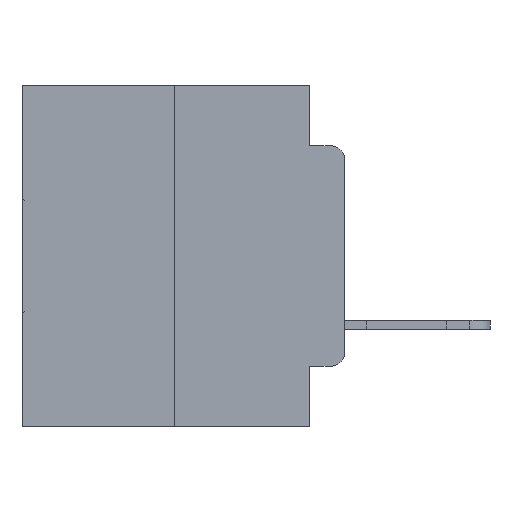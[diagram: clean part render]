
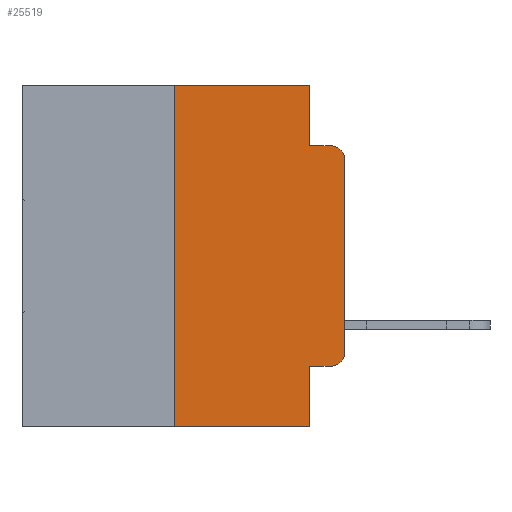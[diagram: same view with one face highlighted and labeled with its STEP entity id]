
A CAD part, left-side view. The second image highlights one B-rep face of the part: STEP entity #25519.
In plain terms, the highlighted planar face has unit normal (-1, 0, 0).
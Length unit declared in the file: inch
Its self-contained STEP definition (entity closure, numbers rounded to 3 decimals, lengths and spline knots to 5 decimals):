
#368 = LINE ( 'NONE', #13695, #17627 ) ;
#556 = VERTEX_POINT ( 'NONE', #14851 ) ;
#1905 = DIRECTION ( 'NONE',  ( 0., 0., 1. ) ) ;
#1913 = DIRECTION ( 'NONE',  ( -1., 0., 0. ) ) ;
#2659 = CARTESIAN_POINT ( 'NONE',  ( 0., 0.473, -0.5 ) ) ;
#3239 = PLANE ( 'NONE',  #23202 ) ;
#3346 = LINE ( 'NONE', #11373, #20342 ) ;
#3619 = CARTESIAN_POINT ( 'NONE',  ( 0., 0.02, -0.0885 ) ) ;
#3624 = EDGE_CURVE ( 'NONE', #8612, #556, #3346, .T. ) ;
#4244 = AXIS2_PLACEMENT_3D ( 'NONE', #15400, #1913, #17586 ) ;
#4437 = EDGE_LOOP ( 'NONE', ( #13223, #20672, #7557, #14636, #18630, #8675, #22464, #27006, #11500, #24499 ) ) ;
#4443 = CARTESIAN_POINT ( 'NONE',  ( 0., 0., -0.3915 ) ) ;
#5061 = DIRECTION ( 'NONE',  ( 0., 0., 1. ) ) ;
#5324 = EDGE_CURVE ( 'NONE', #5730, #9321, #368, .T. ) ;
#5351 = VECTOR ( 'NONE', #17776, 39.37008 ) ;
#5596 = DIRECTION ( 'NONE',  ( 0., 0., -1. ) ) ;
#5730 = VERTEX_POINT ( 'NONE', #14705 ) ;
#6074 = LINE ( 'NONE', #17747, #5351 ) ;
#7419 = CIRCLE ( 'NONE', #11781, 0.02 ) ;
#7557 = ORIENTED_EDGE ( 'NONE', *, *, #8856, .F. ) ;
#7563 = VERTEX_POINT ( 'NONE', #3619 ) ;
#7649 = LINE ( 'NONE', #22081, #18677 ) ;
#8260 = LINE ( 'NONE', #24916, #19264 ) ;
#8612 = VERTEX_POINT ( 'NONE', #14061 ) ;
#8675 = ORIENTED_EDGE ( 'NONE', *, *, #19007, .F. ) ;
#8856 = EDGE_CURVE ( 'NONE', #11102, #7563, #16399, .T. ) ;
#9321 = VERTEX_POINT ( 'NONE', #11405 ) ;
#9778 = EDGE_CURVE ( 'NONE', #556, #11102, #7649, .T. ) ;
#9865 = CARTESIAN_POINT ( 'NONE',  ( 0., 0., -0.1085 ) ) ;
#10668 = VERTEX_POINT ( 'NONE', #4443 ) ;
#11102 = VERTEX_POINT ( 'NONE', #11675 ) ;
#11232 = DIRECTION ( 'NONE',  ( -1., 0., 0. ) ) ;
#11373 = CARTESIAN_POINT ( 'NONE',  ( 0., 0.473, 0. ) ) ;
#11405 = CARTESIAN_POINT ( 'NONE',  ( 0., 0.051, -0.5 ) ) ;
#11500 = ORIENTED_EDGE ( 'NONE', *, *, #11888, .T. ) ;
#11675 = CARTESIAN_POINT ( 'NONE',  ( 0., 0.051, -0.0885 ) ) ;
#11781 = AXIS2_PLACEMENT_3D ( 'NONE', #24346, #11232, #26431 ) ;
#11888 = EDGE_CURVE ( 'NONE', #5730, #21896, #6074, .T. ) ;
#13223 = ORIENTED_EDGE ( 'NONE', *, *, #26983, .T. ) ;
#13494 = VERTEX_POINT ( 'NONE', #15680 ) ;
#13695 = CARTESIAN_POINT ( 'NONE',  ( 0., 0.051, 0. ) ) ;
#13882 = LINE ( 'NONE', #2659, #24120 ) ;
#13913 = DIRECTION ( 'NONE',  ( 0., -1., 0. ) ) ;
#14061 = CARTESIAN_POINT ( 'NONE',  ( 0., 0.25, 0. ) ) ;
#14097 = VECTOR ( 'NONE', #1905, 39.37008 ) ;
#14413 = CARTESIAN_POINT ( 'NONE',  ( 0., 0.02, -0.4115 ) ) ;
#14636 = ORIENTED_EDGE ( 'NONE', *, *, #9778, .F. ) ;
#14705 = CARTESIAN_POINT ( 'NONE',  ( 0., 0.051, -0.4115 ) ) ;
#14851 = CARTESIAN_POINT ( 'NONE',  ( 0., 0.051, 0. ) ) ;
#15393 = CARTESIAN_POINT ( 'NONE',  ( 0., 0., 0. ) ) ;
#15400 = CARTESIAN_POINT ( 'NONE',  ( 0., 0.02, -0.3915 ) ) ;
#15439 = CIRCLE ( 'NONE', #4244, 0.02 ) ;
#15680 = CARTESIAN_POINT ( 'NONE',  ( 0., 0.25, -0.5 ) ) ;
#15879 = FACE_OUTER_BOUND ( 'NONE', #4437, .T. ) ;
#16399 = LINE ( 'NONE', #25986, #22204 ) ;
#17586 = DIRECTION ( 'NONE',  ( 0., 0., -1. ) ) ;
#17627 = VECTOR ( 'NONE', #26081, 39.37008 ) ;
#17747 = CARTESIAN_POINT ( 'NONE',  ( 0., 0.051, -0.4115 ) ) ;
#17776 = DIRECTION ( 'NONE',  ( 0., -1., 0. ) ) ;
#18630 = ORIENTED_EDGE ( 'NONE', *, *, #3624, .F. ) ;
#18677 = VECTOR ( 'NONE', #21985, 39.37008 ) ;
#18781 = DIRECTION ( 'NONE',  ( 1., 0., 0. ) ) ;
#19007 = EDGE_CURVE ( 'NONE', #13494, #8612, #8260, .T. ) ;
#19264 = VECTOR ( 'NONE', #5061, 39.37008 ) ;
#20342 = VECTOR ( 'NONE', #24011, 39.37008 ) ;
#20672 = ORIENTED_EDGE ( 'NONE', *, *, #21274, .T. ) ;
#20707 = DIRECTION ( 'NONE',  ( 0., -1., 0. ) ) ;
#21204 = EDGE_CURVE ( 'NONE', #21896, #10668, #15439, .T. ) ;
#21274 = EDGE_CURVE ( 'NONE', #27935, #7563, #7419, .T. ) ;
#21896 = VERTEX_POINT ( 'NONE', #14413 ) ;
#21985 = DIRECTION ( 'NONE',  ( 0., 0., -1. ) ) ;
#22081 = CARTESIAN_POINT ( 'NONE',  ( 0., 0.051, 0. ) ) ;
#22204 = VECTOR ( 'NONE', #20707, 39.37008 ) ;
#22464 = ORIENTED_EDGE ( 'NONE', *, *, #24164, .T. ) ;
#23202 = AXIS2_PLACEMENT_3D ( 'NONE', #25284, #18781, #5596 ) ;
#24011 = DIRECTION ( 'NONE',  ( 0., -1., 0. ) ) ;
#24120 = VECTOR ( 'NONE', #13913, 39.37008 ) ;
#24164 = EDGE_CURVE ( 'NONE', #13494, #9321, #13882, .T. ) ;
#24346 = CARTESIAN_POINT ( 'NONE',  ( 0., 0.02, -0.1085 ) ) ;
#24499 = ORIENTED_EDGE ( 'NONE', *, *, #21204, .T. ) ;
#24916 = CARTESIAN_POINT ( 'NONE',  ( 0., 0.25, 0. ) ) ;
#25284 = CARTESIAN_POINT ( 'NONE',  ( 0., 0.473, 0. ) ) ;
#25519 = ADVANCED_FACE ( 'NONE', ( #15879 ), #3239, .F. ) ;
#25610 = LINE ( 'NONE', #15393, #14097 ) ;
#25986 = CARTESIAN_POINT ( 'NONE',  ( 0., 0.051, -0.0885 ) ) ;
#26081 = DIRECTION ( 'NONE',  ( 0., 0., -1. ) ) ;
#26431 = DIRECTION ( 'NONE',  ( 0., 0., -1. ) ) ;
#26983 = EDGE_CURVE ( 'NONE', #10668, #27935, #25610, .T. ) ;
#27006 = ORIENTED_EDGE ( 'NONE', *, *, #5324, .F. ) ;
#27935 = VERTEX_POINT ( 'NONE', #9865 ) ;
